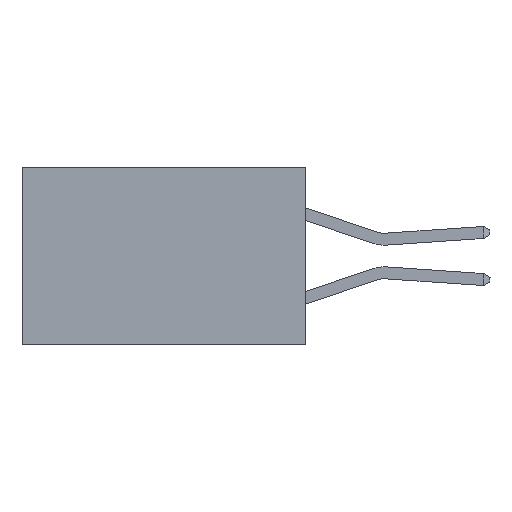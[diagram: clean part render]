
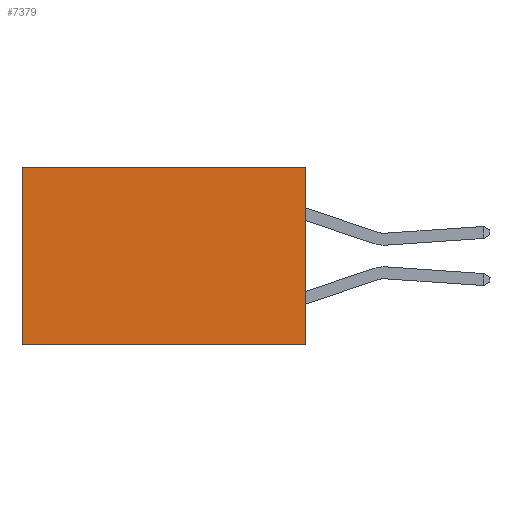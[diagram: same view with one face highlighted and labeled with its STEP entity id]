
A CAD part, left-side view. The second image highlights one B-rep face of the part: STEP entity #7379.
In plain terms, the highlighted planar face has unit normal (-1, 0, 0).
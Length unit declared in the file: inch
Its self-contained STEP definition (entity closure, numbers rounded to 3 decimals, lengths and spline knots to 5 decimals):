
#411 = ORIENTED_EDGE ( 'NONE', *, *, #21169, .F. ) ;
#1565 = VERTEX_POINT ( 'NONE', #18226 ) ;
#1843 = ORIENTED_EDGE ( 'NONE', *, *, #28868, .T. ) ;
#1872 = VERTEX_POINT ( 'NONE', #9899 ) ;
#2612 = CARTESIAN_POINT ( 'NONE',  ( 0.277, 0.59, -0.37 ) ) ;
#2822 = AXIS2_PLACEMENT_3D ( 'NONE', #19708, #19458, #19453 ) ;
#3559 = EDGE_LOOP ( 'NONE', ( #25056, #23880, #411, #1843 ) ) ;
#4145 = CARTESIAN_POINT ( 'NONE',  ( 0.277, 0., -0.37 ) ) ;
#7379 = ADVANCED_FACE ( 'NONE', ( #8129 ), #19519, .F. ) ;
#8129 = FACE_OUTER_BOUND ( 'NONE', #3559, .T. ) ;
#8881 = VECTOR ( 'NONE', #22243, 39.37008 ) ;
#9344 = LINE ( 'NONE', #28911, #28571 ) ;
#9899 = CARTESIAN_POINT ( 'NONE',  ( 0.277, 0.59, -0.37 ) ) ;
#10516 = DIRECTION ( 'NONE',  ( 0., 0., -1. ) ) ;
#10909 = VECTOR ( 'NONE', #10516, 39.37008 ) ;
#11014 = VECTOR ( 'NONE', #31798, 39.37008 ) ;
#11784 = EDGE_CURVE ( 'NONE', #32203, #1872, #30150, .T. ) ;
#16363 = CARTESIAN_POINT ( 'NONE',  ( 0.277, 0.59, 0. ) ) ;
#18226 = CARTESIAN_POINT ( 'NONE',  ( 0.277, 0., 0. ) ) ;
#19453 = DIRECTION ( 'NONE',  ( 0., 0., -1. ) ) ;
#19458 = DIRECTION ( 'NONE',  ( 1., 0., 0. ) ) ;
#19519 = PLANE ( 'NONE',  #2822 ) ;
#19708 = CARTESIAN_POINT ( 'NONE',  ( 0.277, 0., -0.37 ) ) ;
#19724 = CARTESIAN_POINT ( 'NONE',  ( 0.277, 0., 0. ) ) ;
#21169 = EDGE_CURVE ( 'NONE', #1565, #24303, #9344, .T. ) ;
#22243 = DIRECTION ( 'NONE',  ( 0., 1., 0. ) ) ;
#23880 = ORIENTED_EDGE ( 'NONE', *, *, #32310, .F. ) ;
#24303 = VERTEX_POINT ( 'NONE', #4145 ) ;
#24355 = LINE ( 'NONE', #29303, #11014 ) ;
#25056 = ORIENTED_EDGE ( 'NONE', *, *, #11784, .T. ) ;
#28571 = VECTOR ( 'NONE', #31417, 39.37008 ) ;
#28868 = EDGE_CURVE ( 'NONE', #1565, #32203, #28917, .T. ) ;
#28911 = CARTESIAN_POINT ( 'NONE',  ( 0.277, 0., -0.37 ) ) ;
#28917 = LINE ( 'NONE', #19724, #8881 ) ;
#29303 = CARTESIAN_POINT ( 'NONE',  ( 0.277, 0., -0.37 ) ) ;
#30150 = LINE ( 'NONE', #2612, #10909 ) ;
#31417 = DIRECTION ( 'NONE',  ( 0., 0., -1. ) ) ;
#31798 = DIRECTION ( 'NONE',  ( 0., 1., 0. ) ) ;
#32203 = VERTEX_POINT ( 'NONE', #16363 ) ;
#32310 = EDGE_CURVE ( 'NONE', #24303, #1872, #24355, .T. ) ;
